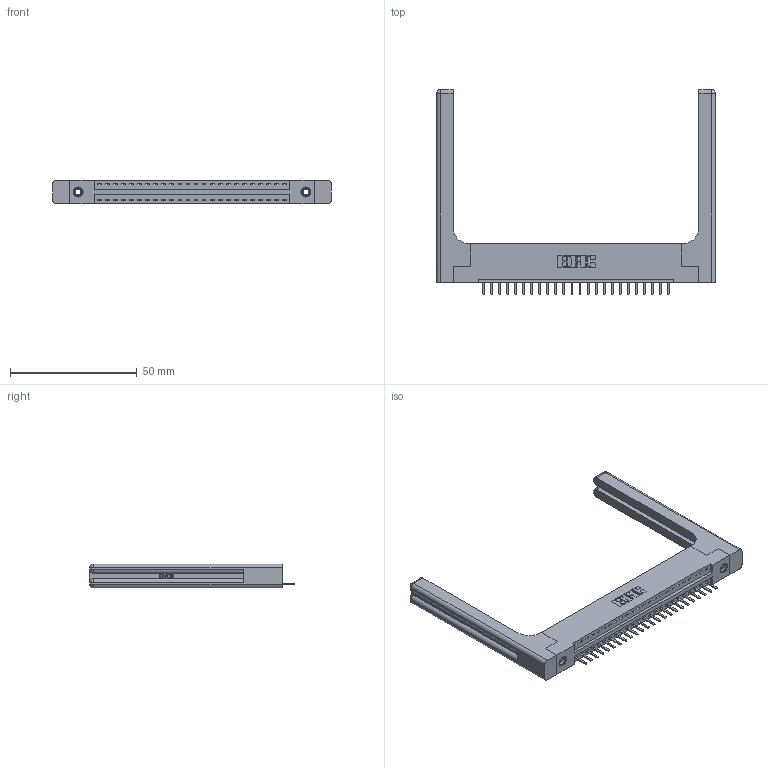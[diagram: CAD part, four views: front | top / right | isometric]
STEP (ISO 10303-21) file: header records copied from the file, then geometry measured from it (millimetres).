
FILE_DESCRIPTION (( 'STEP AP203' ), '1' );
FILE_NAME ('396-024-520-158.STEP', '2019-10-27T05:34:58', ( '' ), ( '' ), 'SwSTEP 2.0', 'SolidWorks 2016', '' );
FILE_SCHEMA (( 'CONFIG_CONTROL_DESIGN' ));
Length unit declared in the file: inch
Products named in the file (5): 396-024-520-158; 345-292-001_345-293-120; 346 Part_Flush Mounting Lugs - 0.156 Dia-TH; 346-220-058_345-220-058; 345-250-001_345-250-001-102
Assembly tree (29 placements, depth 2):
  396-024-520-158
    346 Part_Flush Mounting Lugs - 0.156 Dia-TH
    345-292-001_345-293-120  x24
    345-250-001_345-250-001-102  x2
    346-220-058_345-220-058  x2
Bounding box: 110.26 x 80.98 x 9.4 mm (x, y, z)
Volume: 17879.8 mm3; surface area: 17695.3 mm2
Topology: 29 solids, 29 shells, 1866 faces, 5411 edges, 3522 vertices
Faces by surface type: plane 1232, cylinder 574, bspline 36, cone 12, sphere 8, torus 4
Entity records: 22614 total; most frequent: CARTESIAN_POINT 4873, ORIENTED_EDGE 3616, DIRECTION 3240, EDGE_CURVE 1808, LINE 1484, VECTOR 1484, VERTEX_POINT 1194, AXIS2_PLACEMENT_3D 878
